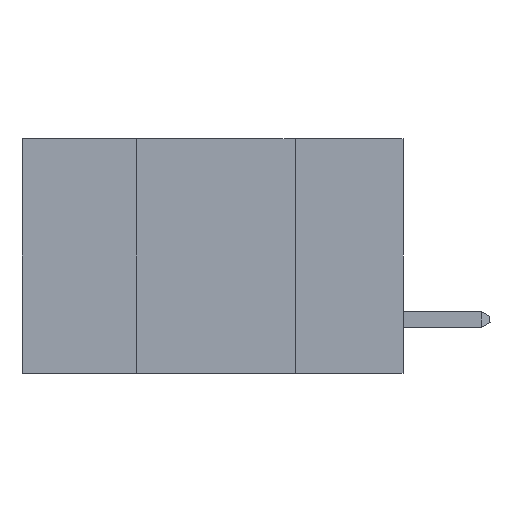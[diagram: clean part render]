
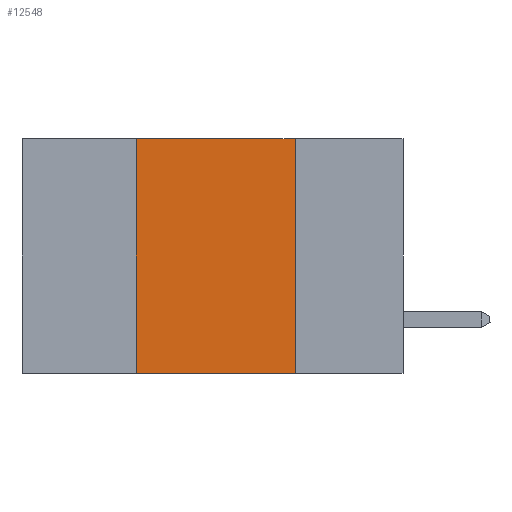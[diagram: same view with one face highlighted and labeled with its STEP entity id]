
A CAD part, left-side view. The second image highlights one B-rep face of the part: STEP entity #12548.
In plain terms, the highlighted planar face has unit normal (-1, 0, 0).
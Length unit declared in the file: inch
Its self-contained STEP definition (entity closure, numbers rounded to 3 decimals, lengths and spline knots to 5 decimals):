
#177 = DIRECTION ( 'NONE',  ( 0., -1., 0. ) ) ;
#1187 = DIRECTION ( 'NONE',  ( 0., -1., 0. ) ) ;
#1250 = EDGE_CURVE ( 'NONE', #13398, #17857, #3108, .T. ) ;
#1412 = VECTOR ( 'NONE', #1187, 39.37008 ) ;
#2043 = CARTESIAN_POINT ( 'NONE',  ( 0., 0.42, -0.37 ) ) ;
#2589 = DIRECTION ( 'NONE',  ( 0., 0., -1. ) ) ;
#3108 = LINE ( 'NONE', #6736, #1412 ) ;
#3440 = VERTEX_POINT ( 'NONE', #2043 ) ;
#4900 = CARTESIAN_POINT ( 'NONE',  ( 0., 0.42, 0. ) ) ;
#5229 = VECTOR ( 'NONE', #2589, 39.37008 ) ;
#5292 = VERTEX_POINT ( 'NONE', #8077 ) ;
#5864 = LINE ( 'NONE', #9545, #17583 ) ;
#6736 = CARTESIAN_POINT ( 'NONE',  ( 0., 0.6, 0. ) ) ;
#6891 = DIRECTION ( 'NONE',  ( 1., 0., 0. ) ) ;
#7224 = EDGE_CURVE ( 'NONE', #17857, #5292, #9288, .T. ) ;
#8077 = CARTESIAN_POINT ( 'NONE',  ( 0., 0.17, -0.37 ) ) ;
#8113 = ORIENTED_EDGE ( 'NONE', *, *, #9150, .T. ) ;
#9150 = EDGE_CURVE ( 'NONE', #3440, #5292, #5864, .T. ) ;
#9288 = LINE ( 'NONE', #9793, #5229 ) ;
#9413 = LINE ( 'NONE', #4900, #12848 ) ;
#9545 = CARTESIAN_POINT ( 'NONE',  ( 0., 0.6, -0.37 ) ) ;
#9793 = CARTESIAN_POINT ( 'NONE',  ( 0., 0.17, 0. ) ) ;
#10281 = ORIENTED_EDGE ( 'NONE', *, *, #15408, .F. ) ;
#11011 = EDGE_LOOP ( 'NONE', ( #14551, #14403, #10281, #8113 ) ) ;
#11648 = CARTESIAN_POINT ( 'NONE',  ( 0., 0.17, 0. ) ) ;
#11969 = AXIS2_PLACEMENT_3D ( 'NONE', #18492, #6891, #17142 ) ;
#12079 = CARTESIAN_POINT ( 'NONE',  ( 0., 0.42, 0. ) ) ;
#12548 = ADVANCED_FACE ( 'NONE', ( #15002 ), #15720, .F. ) ;
#12848 = VECTOR ( 'NONE', #13859, 39.37008 ) ;
#13398 = VERTEX_POINT ( 'NONE', #12079 ) ;
#13859 = DIRECTION ( 'NONE',  ( 0., 0., 1. ) ) ;
#14403 = ORIENTED_EDGE ( 'NONE', *, *, #1250, .F. ) ;
#14551 = ORIENTED_EDGE ( 'NONE', *, *, #7224, .F. ) ;
#15002 = FACE_OUTER_BOUND ( 'NONE', #11011, .T. ) ;
#15408 = EDGE_CURVE ( 'NONE', #3440, #13398, #9413, .T. ) ;
#15720 = PLANE ( 'NONE',  #11969 ) ;
#17142 = DIRECTION ( 'NONE',  ( 0., 0., -1. ) ) ;
#17583 = VECTOR ( 'NONE', #177, 39.37008 ) ;
#17857 = VERTEX_POINT ( 'NONE', #11648 ) ;
#18492 = CARTESIAN_POINT ( 'NONE',  ( 0., 0.6, 0. ) ) ;
